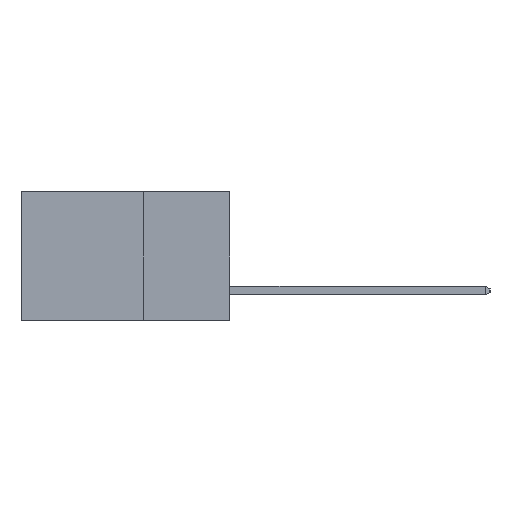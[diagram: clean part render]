
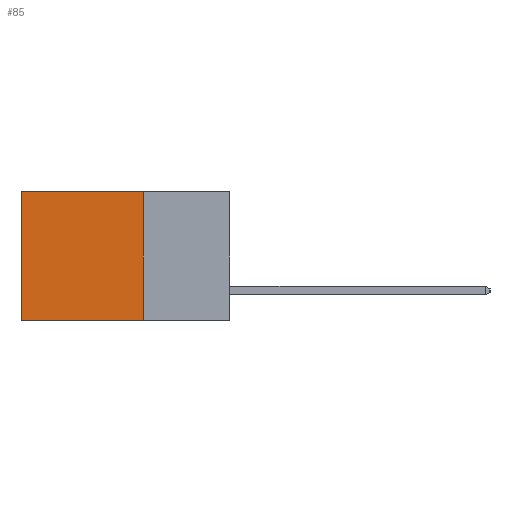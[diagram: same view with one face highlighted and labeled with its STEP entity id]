
A CAD part, left-side view. The second image highlights one B-rep face of the part: STEP entity #85.
In plain terms, the highlighted planar face has unit normal (-1, 0, 0).
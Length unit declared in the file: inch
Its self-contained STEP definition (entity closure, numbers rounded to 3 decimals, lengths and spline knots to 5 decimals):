
#85 = ADVANCED_FACE ( 'NONE', ( #3610 ), #1140, .F. ) ;
#584 = CARTESIAN_POINT ( 'NONE',  ( 0.2615, 0.25, -0.37 ) ) ;
#787 = LINE ( 'NONE', #3626, #7030 ) ;
#1023 = EDGE_CURVE ( 'NONE', #6206, #10946, #9186, .T. ) ;
#1138 = CARTESIAN_POINT ( 'NONE',  ( 0.2615, 0.25, -0.37 ) ) ;
#1140 = PLANE ( 'NONE',  #3842 ) ;
#1286 = LINE ( 'NONE', #584, #7897 ) ;
#1843 = DIRECTION ( 'NONE',  ( 0., 0., -1. ) ) ;
#2126 = CARTESIAN_POINT ( 'NONE',  ( 0.2615, 0.25, -0.37 ) ) ;
#2343 = ORIENTED_EDGE ( 'NONE', *, *, #12460, .F. ) ;
#3339 = ORIENTED_EDGE ( 'NONE', *, *, #8643, .F. ) ;
#3610 = FACE_OUTER_BOUND ( 'NONE', #10501, .T. ) ;
#3626 = CARTESIAN_POINT ( 'NONE',  ( 0.2615, 0.25, -0.37 ) ) ;
#3842 = AXIS2_PLACEMENT_3D ( 'NONE', #1138, #4419, #7182 ) ;
#3982 = CARTESIAN_POINT ( 'NONE',  ( 0.2615, 0.6, -0.37 ) ) ;
#4419 = DIRECTION ( 'NONE',  ( 1., 0., 0. ) ) ;
#4611 = CARTESIAN_POINT ( 'NONE',  ( 0.2615, 0.25, 0. ) ) ;
#4897 = DIRECTION ( 'NONE',  ( 0., 1., 0. ) ) ;
#5433 = ORIENTED_EDGE ( 'NONE', *, *, #1023, .T. ) ;
#6163 = VERTEX_POINT ( 'NONE', #15270 ) ;
#6206 = VERTEX_POINT ( 'NONE', #12983 ) ;
#7030 = VECTOR ( 'NONE', #4897, 39.37008 ) ;
#7182 = DIRECTION ( 'NONE',  ( 0., 0., -1. ) ) ;
#7897 = VECTOR ( 'NONE', #1843, 39.37008 ) ;
#8643 = EDGE_CURVE ( 'NONE', #6163, #10832, #1286, .T. ) ;
#9139 = LINE ( 'NONE', #4611, #15726 ) ;
#9186 = LINE ( 'NONE', #3982, #15773 ) ;
#10501 = EDGE_LOOP ( 'NONE', ( #5433, #2343, #3339, #11661 ) ) ;
#10832 = VERTEX_POINT ( 'NONE', #2126 ) ;
#10946 = VERTEX_POINT ( 'NONE', #13576 ) ;
#11661 = ORIENTED_EDGE ( 'NONE', *, *, #12964, .T. ) ;
#12460 = EDGE_CURVE ( 'NONE', #10832, #10946, #787, .T. ) ;
#12964 = EDGE_CURVE ( 'NONE', #6163, #6206, #9139, .T. ) ;
#12983 = CARTESIAN_POINT ( 'NONE',  ( 0.2615, 0.6, 0. ) ) ;
#13576 = CARTESIAN_POINT ( 'NONE',  ( 0.2615, 0.6, -0.37 ) ) ;
#14484 = DIRECTION ( 'NONE',  ( 0., 1., 0. ) ) ;
#15133 = DIRECTION ( 'NONE',  ( 0., 0., -1. ) ) ;
#15270 = CARTESIAN_POINT ( 'NONE',  ( 0.2615, 0.25, 0. ) ) ;
#15726 = VECTOR ( 'NONE', #14484, 39.37008 ) ;
#15773 = VECTOR ( 'NONE', #15133, 39.37008 ) ;
